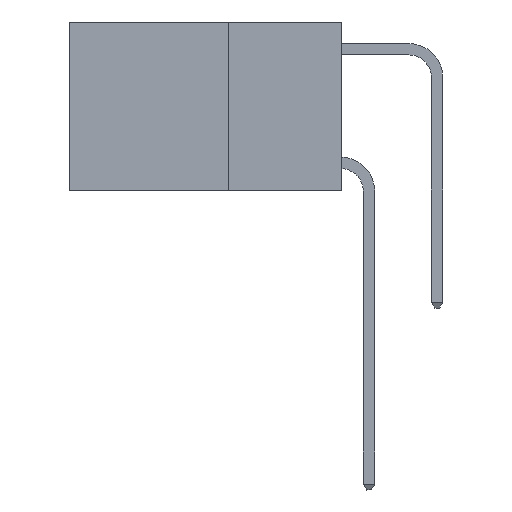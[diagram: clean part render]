
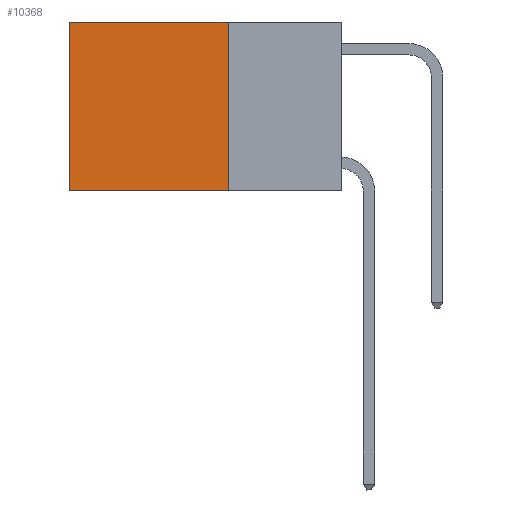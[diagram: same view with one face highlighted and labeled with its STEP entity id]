
A CAD part, left-side view. The second image highlights one B-rep face of the part: STEP entity #10368.
In plain terms, the highlighted planar face has unit normal (-1, 0, 0).
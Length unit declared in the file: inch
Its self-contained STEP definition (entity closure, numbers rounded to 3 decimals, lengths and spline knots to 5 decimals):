
#16 = DIRECTION ( 'NONE',  ( 0., 1., 0. ) ) ;
#285 = CARTESIAN_POINT ( 'NONE',  ( 0.2625, 0.25, 0. ) ) ;
#993 = VECTOR ( 'NONE', #17421, 39.37008 ) ;
#1317 = LINE ( 'NONE', #1554, #2810 ) ;
#1554 = CARTESIAN_POINT ( 'NONE',  ( 0.2625, 0.6, 0. ) ) ;
#2810 = VECTOR ( 'NONE', #21453, 39.37008 ) ;
#2858 = VECTOR ( 'NONE', #13115, 39.37008 ) ;
#4141 = CARTESIAN_POINT ( 'NONE',  ( 0.2625, 0.6, 0. ) ) ;
#4635 = CARTESIAN_POINT ( 'NONE',  ( 0.2625, 0.25, -0.37 ) ) ;
#5577 = PLANE ( 'NONE',  #22670 ) ;
#7247 = EDGE_CURVE ( 'NONE', #19018, #19659, #20038, .T. ) ;
#7963 = DIRECTION ( 'NONE',  ( 1., 0., 0. ) ) ;
#8317 = ORIENTED_EDGE ( 'NONE', *, *, #7247, .F. ) ;
#8591 = EDGE_CURVE ( 'NONE', #12125, #19018, #11202, .T. ) ;
#9150 = CARTESIAN_POINT ( 'NONE',  ( 0.2625, 0.25, -0.37 ) ) ;
#9935 = EDGE_CURVE ( 'NONE', #20503, #19659, #1317, .T. ) ;
#10109 = LINE ( 'NONE', #12143, #993 ) ;
#10313 = ORIENTED_EDGE ( 'NONE', *, *, #8591, .F. ) ;
#10368 = ADVANCED_FACE ( 'NONE', ( #16739 ), #5577, .F. ) ;
#11180 = CARTESIAN_POINT ( 'NONE',  ( 0.2625, 0.6, -0.37 ) ) ;
#11202 = LINE ( 'NONE', #11551, #2858 ) ;
#11551 = CARTESIAN_POINT ( 'NONE',  ( 0.2625, 0.25, 0. ) ) ;
#11931 = VECTOR ( 'NONE', #16, 39.37008 ) ;
#12125 = VERTEX_POINT ( 'NONE', #16027 ) ;
#12143 = CARTESIAN_POINT ( 'NONE',  ( 0.2625, 0.25, 0. ) ) ;
#12291 = EDGE_CURVE ( 'NONE', #12125, #20503, #10109, .T. ) ;
#13115 = DIRECTION ( 'NONE',  ( 0., 0., -1. ) ) ;
#16009 = ORIENTED_EDGE ( 'NONE', *, *, #9935, .T. ) ;
#16027 = CARTESIAN_POINT ( 'NONE',  ( 0.2625, 0.25, 0. ) ) ;
#16739 = FACE_OUTER_BOUND ( 'NONE', #17290, .T. ) ;
#17290 = EDGE_LOOP ( 'NONE', ( #16009, #8317, #10313, #22013 ) ) ;
#17421 = DIRECTION ( 'NONE',  ( 0., 1., 0. ) ) ;
#18867 = DIRECTION ( 'NONE',  ( 0., 0., -1. ) ) ;
#19018 = VERTEX_POINT ( 'NONE', #4635 ) ;
#19659 = VERTEX_POINT ( 'NONE', #11180 ) ;
#20038 = LINE ( 'NONE', #9150, #11931 ) ;
#20503 = VERTEX_POINT ( 'NONE', #4141 ) ;
#21453 = DIRECTION ( 'NONE',  ( 0., 0., -1. ) ) ;
#22013 = ORIENTED_EDGE ( 'NONE', *, *, #12291, .T. ) ;
#22670 = AXIS2_PLACEMENT_3D ( 'NONE', #285, #7963, #18867 ) ;
